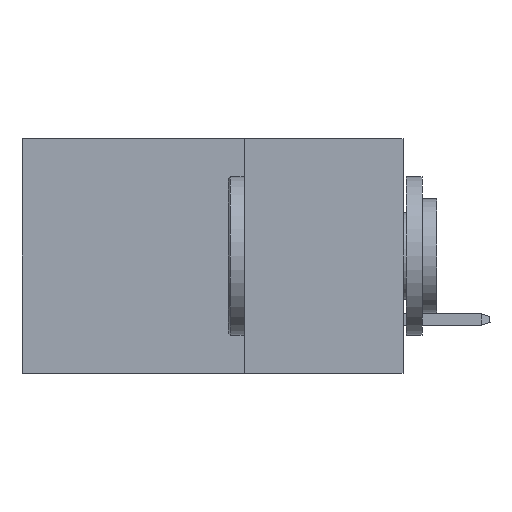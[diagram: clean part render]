
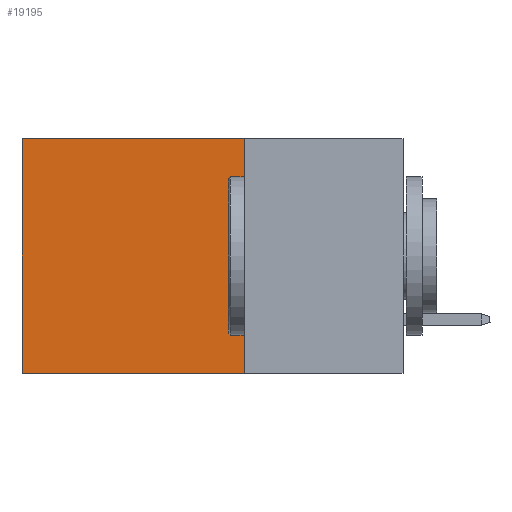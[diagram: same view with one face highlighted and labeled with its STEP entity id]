
A CAD part, left-side view. The second image highlights one B-rep face of the part: STEP entity #19195.
In plain terms, the highlighted planar face has unit normal (-1, 0, 0).
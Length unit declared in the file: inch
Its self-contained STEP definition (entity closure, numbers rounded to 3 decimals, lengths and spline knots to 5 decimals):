
#737 = CARTESIAN_POINT ( 'NONE',  ( 0.2875, 0.25, 0. ) ) ;
#6878 = VECTOR ( 'NONE', #31020, 39.37008 ) ;
#8370 = EDGE_CURVE ( 'NONE', #35095, #10060, #9330, .T. ) ;
#9072 = ORIENTED_EDGE ( 'NONE', *, *, #8370, .F. ) ;
#9330 = LINE ( 'NONE', #11479, #6878 ) ;
#10060 = VERTEX_POINT ( 'NONE', #20154 ) ;
#11479 = CARTESIAN_POINT ( 'NONE',  ( 0.2875, 0.25, -0.37 ) ) ;
#11802 = EDGE_LOOP ( 'NONE', ( #23991, #9072, #20447, #34564 ) ) ;
#12293 = CARTESIAN_POINT ( 'NONE',  ( 0.2875, 0.25, 0. ) ) ;
#13742 = VECTOR ( 'NONE', #28873, 39.37008 ) ;
#14067 = CARTESIAN_POINT ( 'NONE',  ( 0.2875, 0.6, 0. ) ) ;
#14772 = VERTEX_POINT ( 'NONE', #26546 ) ;
#15218 = CARTESIAN_POINT ( 'NONE',  ( 0.2875, 0.25, 0. ) ) ;
#16192 = DIRECTION ( 'NONE',  ( 1., 0., 0. ) ) ;
#16583 = LINE ( 'NONE', #14067, #27643 ) ;
#17847 = LINE ( 'NONE', #12293, #22235 ) ;
#18863 = FACE_OUTER_BOUND ( 'NONE', #11802, .T. ) ;
#19195 = ADVANCED_FACE ( 'NONE', ( #18863 ), #24595, .F. ) ;
#19883 = VERTEX_POINT ( 'NONE', #15218 ) ;
#20154 = CARTESIAN_POINT ( 'NONE',  ( 0.2875, 0.6, -0.37 ) ) ;
#20447 = ORIENTED_EDGE ( 'NONE', *, *, #31518, .F. ) ;
#22235 = VECTOR ( 'NONE', #34507, 39.37008 ) ;
#23991 = ORIENTED_EDGE ( 'NONE', *, *, #34477, .T. ) ;
#24595 = PLANE ( 'NONE',  #34032 ) ;
#25285 = LINE ( 'NONE', #737, #13742 ) ;
#26011 = EDGE_CURVE ( 'NONE', #19883, #14772, #17847, .T. ) ;
#26546 = CARTESIAN_POINT ( 'NONE',  ( 0.2875, 0.6, 0. ) ) ;
#27643 = VECTOR ( 'NONE', #28050, 39.37008 ) ;
#28050 = DIRECTION ( 'NONE',  ( 0., 0., -1. ) ) ;
#28189 = CARTESIAN_POINT ( 'NONE',  ( 0.2875, 0.25, -0.37 ) ) ;
#28873 = DIRECTION ( 'NONE',  ( 0., 0., -1. ) ) ;
#29815 = CARTESIAN_POINT ( 'NONE',  ( 0.2875, 0.25, 0. ) ) ;
#31020 = DIRECTION ( 'NONE',  ( 0., 1., 0. ) ) ;
#31518 = EDGE_CURVE ( 'NONE', #19883, #35095, #25285, .T. ) ;
#33035 = DIRECTION ( 'NONE',  ( 0., 0., -1. ) ) ;
#34032 = AXIS2_PLACEMENT_3D ( 'NONE', #29815, #16192, #33035 ) ;
#34477 = EDGE_CURVE ( 'NONE', #14772, #10060, #16583, .T. ) ;
#34507 = DIRECTION ( 'NONE',  ( 0., 1., 0. ) ) ;
#34564 = ORIENTED_EDGE ( 'NONE', *, *, #26011, .T. ) ;
#35095 = VERTEX_POINT ( 'NONE', #28189 ) ;
